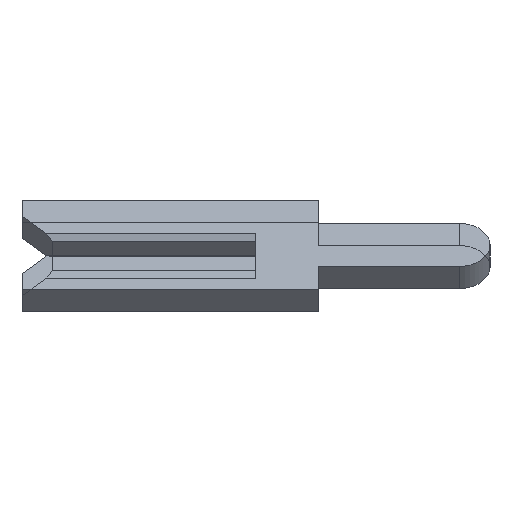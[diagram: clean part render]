
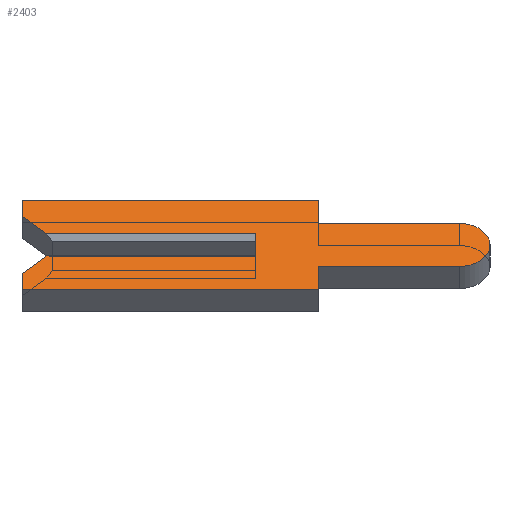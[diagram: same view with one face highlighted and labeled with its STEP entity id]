
A CAD part, left-side view. The second image highlights one B-rep face of the part: STEP entity #2403.
In plain terms, the highlighted face is planar.
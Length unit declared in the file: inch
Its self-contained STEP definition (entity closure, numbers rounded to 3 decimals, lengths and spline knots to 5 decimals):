
#19 = DIRECTION ( 'NONE',  ( 0., 0., -1. ) ) ;
#36 = ORIENTED_EDGE ( 'NONE', *, *, #251, .F. ) ;
#121 = LINE ( 'NONE', #2602, #1555 ) ;
#201 = DIRECTION ( 'NONE',  ( 0., 1., 0. ) ) ;
#251 = EDGE_CURVE ( 'NONE', #3024, #1564, #3064, .T. ) ;
#270 = DIRECTION ( 'NONE',  ( 0., -1., 0. ) ) ;
#304 = EDGE_CURVE ( 'NONE', #1801, #3321, #580, .T. ) ;
#327 = LINE ( 'NONE', #2759, #2121 ) ;
#376 = VECTOR ( 'NONE', #2530, 39.37008 ) ;
#409 = LINE ( 'NONE', #2249, #2457 ) ;
#413 = ORIENTED_EDGE ( 'NONE', *, *, #1954, .F. ) ;
#419 = ORIENTED_EDGE ( 'NONE', *, *, #2488, .F. ) ;
#422 = CARTESIAN_POINT ( 'NONE',  ( -0.01, 0.15, 0.01 ) ) ;
#432 = EDGE_CURVE ( 'NONE', #460, #3073, #1354, .T. ) ;
#460 = VERTEX_POINT ( 'NONE', #787 ) ;
#513 = CARTESIAN_POINT ( 'NONE',  ( -0.01, -0.1305, -0.01 ) ) ;
#540 = VERTEX_POINT ( 'NONE', #2870 ) ;
#543 = EDGE_CURVE ( 'NONE', #540, #3108, #1790, .T. ) ;
#573 = CARTESIAN_POINT ( 'NONE',  ( -0.01, 0.15, 0.04 ) ) ;
#575 = LINE ( 'NONE', #573, #613 ) ;
#580 = LINE ( 'NONE', #2241, #997 ) ;
#613 = VECTOR ( 'NONE', #270, 39.37008 ) ;
#625 = VERTEX_POINT ( 'NONE', #1370 ) ;
#700 = CARTESIAN_POINT ( 'NONE',  ( -0.01, 0.1305, 0.0065 ) ) ;
#721 = CARTESIAN_POINT ( 'NONE',  ( -0.01, 0.15, -0.04 ) ) ;
#746 = VERTEX_POINT ( 'NONE', #1349 ) ;
#773 = CARTESIAN_POINT ( 'NONE',  ( -0.01, -0.1305, 0. ) ) ;
#787 = CARTESIAN_POINT ( 'NONE',  ( -0.01, -0.1305, 0.0195 ) ) ;
#796 = ORIENTED_EDGE ( 'NONE', *, *, #304, .F. ) ;
#902 = CARTESIAN_POINT ( 'NONE',  ( -0.01, -0.04, -0.04 ) ) ;
#959 = DIRECTION ( 'NONE',  ( 0., 0., -1. ) ) ;
#997 = VECTOR ( 'NONE', #1472, 39.37008 ) ;
#998 = LINE ( 'NONE', #2623, #1870 ) ;
#999 = VERTEX_POINT ( 'NONE', #2204 ) ;
#1033 = ORIENTED_EDGE ( 'NONE', *, *, #432, .F. ) ;
#1035 = VECTOR ( 'NONE', #2285, 39.37008 ) ;
#1110 = LINE ( 'NONE', #422, #376 ) ;
#1149 = CARTESIAN_POINT ( 'NONE',  ( -0.01, 0., -0.01 ) ) ;
#1153 = ORIENTED_EDGE ( 'NONE', *, *, #2174, .F. ) ;
#1223 = AXIS2_PLACEMENT_3D ( 'NONE', #773, #1318, #1565 ) ;
#1243 = DIRECTION ( 'NONE',  ( 0., 0., 1. ) ) ;
#1267 = CARTESIAN_POINT ( 'NONE',  ( -0.01, 0.15, 0.04 ) ) ;
#1274 = ORIENTED_EDGE ( 'NONE', *, *, #2163, .F. ) ;
#1278 = DIRECTION ( 'NONE',  ( 0., -1., 0. ) ) ;
#1309 = CARTESIAN_POINT ( 'NONE',  ( -0.01, 0.15, 0.026 ) ) ;
#1318 = DIRECTION ( 'NONE',  ( 1., 0., 0. ) ) ;
#1346 = CARTESIAN_POINT ( 'NONE',  ( -0.01, -0.04, -0.0195 ) ) ;
#1347 = CARTESIAN_POINT ( 'NONE',  ( -0.01, 0.134, -0.01 ) ) ;
#1349 = CARTESIAN_POINT ( 'NONE',  ( -0.01, -0.04, 0.04 ) ) ;
#1354 = CIRCLE ( 'NONE', #1223, 0.0195 ) ;
#1370 = CARTESIAN_POINT ( 'NONE',  ( -0.01, 0., 0.01 ) ) ;
#1438 = FACE_OUTER_BOUND ( 'NONE', #2661, .T. ) ;
#1472 = DIRECTION ( 'NONE',  ( 0., -0.707, 0.707 ) ) ;
#1477 = LINE ( 'NONE', #721, #1035 ) ;
#1501 = DIRECTION ( 'NONE',  ( 0., 0.707, 0.707 ) ) ;
#1520 = VECTOR ( 'NONE', #201, 39.37008 ) ;
#1544 = ORIENTED_EDGE ( 'NONE', *, *, #2748, .F. ) ;
#1555 = VECTOR ( 'NONE', #1243, 39.37008 ) ;
#1564 = VERTEX_POINT ( 'NONE', #902 ) ;
#1565 = DIRECTION ( 'NONE',  ( 0., 0., -1. ) ) ;
#1632 = AXIS2_PLACEMENT_3D ( 'NONE', #2514, #2003, #959 ) ;
#1702 = CARTESIAN_POINT ( 'NONE',  ( -0.01, 0.15, -0.04 ) ) ;
#1738 = CARTESIAN_POINT ( 'NONE',  ( -0.01, -0.1305, -0.0195 ) ) ;
#1767 = ORIENTED_EDGE ( 'NONE', *, *, #2360, .T. ) ;
#1790 = LINE ( 'NONE', #1309, #3103 ) ;
#1801 = VERTEX_POINT ( 'NONE', #2997 ) ;
#1815 = VERTEX_POINT ( 'NONE', #1149 ) ;
#1867 = DIRECTION ( 'NONE',  ( 0., 0., 1. ) ) ;
#1870 = VECTOR ( 'NONE', #19, 39.37008 ) ;
#1954 = EDGE_CURVE ( 'NONE', #1564, #2135, #1477, .T. ) ;
#1963 = ORIENTED_EDGE ( 'NONE', *, *, #3233, .F. ) ;
#1964 = DIRECTION ( 'NONE',  ( 0., -1., 0. ) ) ;
#2003 = DIRECTION ( 'NONE',  ( 1., 0., 0. ) ) ;
#2121 = VECTOR ( 'NONE', #2783, 39.37008 ) ;
#2135 = VERTEX_POINT ( 'NONE', #1702 ) ;
#2161 = VECTOR ( 'NONE', #1278, 39.37008 ) ;
#2163 = EDGE_CURVE ( 'NONE', #999, #540, #2654, .T. ) ;
#2174 = EDGE_CURVE ( 'NONE', #2859, #460, #409, .T. ) ;
#2196 = ORIENTED_EDGE ( 'NONE', *, *, #2819, .F. ) ;
#2204 = CARTESIAN_POINT ( 'NONE',  ( -0.01, 0.134, 0.01 ) ) ;
#2241 = CARTESIAN_POINT ( 'NONE',  ( -0.01, 0.1305, -0.0065 ) ) ;
#2247 = LINE ( 'NONE', #3049, #1520 ) ;
#2249 = CARTESIAN_POINT ( 'NONE',  ( -0.01, -0.04, 0.0195 ) ) ;
#2285 = DIRECTION ( 'NONE',  ( 0., 1., 0. ) ) ;
#2295 = CARTESIAN_POINT ( 'NONE',  ( -0.01, -0.04, 0.0195 ) ) ;
#2360 = EDGE_CURVE ( 'NONE', #999, #625, #1110, .T. ) ;
#2403 = ADVANCED_FACE ( 'NONE', ( #1438 ), #3025, .F. ) ;
#2412 = LINE ( 'NONE', #513, #2161 ) ;
#2420 = EDGE_CURVE ( 'NONE', #1815, #625, #327, .T. ) ;
#2431 = ORIENTED_EDGE ( 'NONE', *, *, #543, .F. ) ;
#2457 = VECTOR ( 'NONE', #1964, 39.37008 ) ;
#2488 = EDGE_CURVE ( 'NONE', #3073, #3024, #2247, .T. ) ;
#2501 = CARTESIAN_POINT ( 'NONE',  ( -0.01, -0.04, -0.04 ) ) ;
#2514 = CARTESIAN_POINT ( 'NONE',  ( -0.01, -0.1305, 0. ) ) ;
#2530 = DIRECTION ( 'NONE',  ( 0., -1., 0. ) ) ;
#2541 = VECTOR ( 'NONE', #2765, 39.37008 ) ;
#2602 = CARTESIAN_POINT ( 'NONE',  ( -0.01, 0.15, -0.026 ) ) ;
#2623 = CARTESIAN_POINT ( 'NONE',  ( -0.01, -0.04, 0.04 ) ) ;
#2654 = LINE ( 'NONE', #700, #3066 ) ;
#2661 = EDGE_LOOP ( 'NONE', ( #1767, #2692, #1544, #796, #2196, #413, #36, #419, #1033, #1153, #1963, #3282, #2431, #1274 ) ) ;
#2692 = ORIENTED_EDGE ( 'NONE', *, *, #2420, .F. ) ;
#2748 = EDGE_CURVE ( 'NONE', #3321, #1815, #2412, .T. ) ;
#2759 = CARTESIAN_POINT ( 'NONE',  ( -0.01, 0., 0.0065 ) ) ;
#2765 = DIRECTION ( 'NONE',  ( 0., 0., -1. ) ) ;
#2783 = DIRECTION ( 'NONE',  ( 0., 0., 1. ) ) ;
#2819 = EDGE_CURVE ( 'NONE', #2135, #1801, #121, .T. ) ;
#2859 = VERTEX_POINT ( 'NONE', #2295 ) ;
#2870 = CARTESIAN_POINT ( 'NONE',  ( -0.01, 0.15, 0.026 ) ) ;
#2997 = CARTESIAN_POINT ( 'NONE',  ( -0.01, 0.15, -0.026 ) ) ;
#3024 = VERTEX_POINT ( 'NONE', #1346 ) ;
#3025 = PLANE ( 'NONE',  #1632 ) ;
#3049 = CARTESIAN_POINT ( 'NONE',  ( -0.01, -0.04, -0.0195 ) ) ;
#3064 = LINE ( 'NONE', #2501, #2541 ) ;
#3066 = VECTOR ( 'NONE', #1501, 39.37008 ) ;
#3073 = VERTEX_POINT ( 'NONE', #1738 ) ;
#3103 = VECTOR ( 'NONE', #1867, 39.37008 ) ;
#3108 = VERTEX_POINT ( 'NONE', #1267 ) ;
#3233 = EDGE_CURVE ( 'NONE', #746, #2859, #998, .T. ) ;
#3282 = ORIENTED_EDGE ( 'NONE', *, *, #3298, .F. ) ;
#3298 = EDGE_CURVE ( 'NONE', #3108, #746, #575, .T. ) ;
#3321 = VERTEX_POINT ( 'NONE', #1347 ) ;
